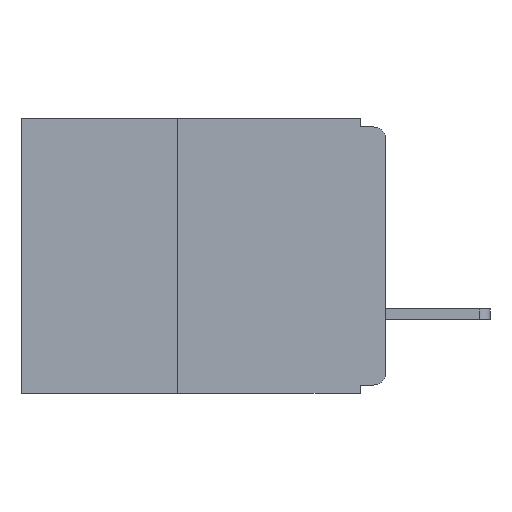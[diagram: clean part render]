
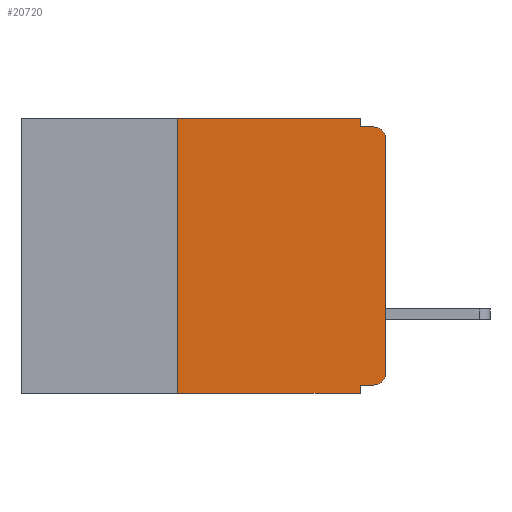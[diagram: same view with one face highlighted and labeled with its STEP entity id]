
A CAD part, left-side view. The second image highlights one B-rep face of the part: STEP entity #20720.
In plain terms, the highlighted planar face has unit normal (-1, 0, 0).
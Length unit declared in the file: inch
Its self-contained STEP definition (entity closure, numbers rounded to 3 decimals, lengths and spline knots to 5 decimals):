
#39 = CARTESIAN_POINT ( 'NONE',  ( 0., 0.031, -0.32 ) ) ;
#455 = ORIENTED_EDGE ( 'NONE', *, *, #13038, .T. ) ;
#470 = CIRCLE ( 'NONE', #14085, 0.015 ) ;
#576 = ORIENTED_EDGE ( 'NONE', *, *, #14436, .F. ) ;
#778 = VERTEX_POINT ( 'NONE', #17617 ) ;
#1560 = DIRECTION ( 'NONE',  ( 1., 0., 0. ) ) ;
#2239 = DIRECTION ( 'NONE',  ( 0., -1., 0. ) ) ;
#2416 = VECTOR ( 'NONE', #14217, 39.37008 ) ;
#2680 = VECTOR ( 'NONE', #23399, 39.37008 ) ;
#3169 = ORIENTED_EDGE ( 'NONE', *, *, #25854, .F. ) ;
#4152 = EDGE_LOOP ( 'NONE', ( #12530, #17470, #6061, #576, #20243, #14952, #4590, #7524, #3169, #455 ) ) ;
#4590 = ORIENTED_EDGE ( 'NONE', *, *, #21514, .T. ) ;
#5326 = CARTESIAN_POINT ( 'NONE',  ( 0., 0.031, -0.01 ) ) ;
#6061 = ORIENTED_EDGE ( 'NONE', *, *, #19302, .F. ) ;
#6496 = EDGE_CURVE ( 'NONE', #16651, #16271, #28083, .T. ) ;
#6736 = EDGE_CURVE ( 'NONE', #778, #7123, #470, .T. ) ;
#7123 = VERTEX_POINT ( 'NONE', #18079 ) ;
#7524 = ORIENTED_EDGE ( 'NONE', *, *, #6496, .F. ) ;
#7761 = VECTOR ( 'NONE', #26527, 39.37008 ) ;
#7963 = DIRECTION ( 'NONE',  ( 0., 0., -1. ) ) ;
#8471 = CARTESIAN_POINT ( 'NONE',  ( 0., 0., -0.01 ) ) ;
#8475 = EDGE_CURVE ( 'NONE', #19391, #31852, #27575, .T. ) ;
#8535 = CARTESIAN_POINT ( 'NONE',  ( 0., 0.015, -0.32 ) ) ;
#8830 = CARTESIAN_POINT ( 'NONE',  ( 0., 0.015, -0.305 ) ) ;
#8921 = CARTESIAN_POINT ( 'NONE',  ( 0., 0.015, -0.025 ) ) ;
#9247 = CARTESIAN_POINT ( 'NONE',  ( 0., 0., 0. ) ) ;
#9705 = CARTESIAN_POINT ( 'NONE',  ( 0., 0.25, 0. ) ) ;
#11346 = DIRECTION ( 'NONE',  ( 0., 0., -1. ) ) ;
#11425 = DIRECTION ( 'NONE',  ( 0., 0., -1. ) ) ;
#12138 = CARTESIAN_POINT ( 'NONE',  ( 0., 0., -0.305 ) ) ;
#12447 = LINE ( 'NONE', #29441, #24897 ) ;
#12530 = ORIENTED_EDGE ( 'NONE', *, *, #26299, .T. ) ;
#13038 = EDGE_CURVE ( 'NONE', #31084, #28289, #14457, .T. ) ;
#14085 = AXIS2_PLACEMENT_3D ( 'NONE', #8921, #26303, #11425 ) ;
#14217 = DIRECTION ( 'NONE',  ( 0., 0., 1. ) ) ;
#14436 = EDGE_CURVE ( 'NONE', #26200, #24440, #17128, .T. ) ;
#14457 = CIRCLE ( 'NONE', #27734, 0.015 ) ;
#14730 = DIRECTION ( 'NONE',  ( 0., -1., 0. ) ) ;
#14875 = LINE ( 'NONE', #29596, #21638 ) ;
#14952 = ORIENTED_EDGE ( 'NONE', *, *, #8475, .F. ) ;
#16020 = CARTESIAN_POINT ( 'NONE',  ( 0., 0.031, 0. ) ) ;
#16253 = AXIS2_PLACEMENT_3D ( 'NONE', #16438, #1560, #19012 ) ;
#16255 = CARTESIAN_POINT ( 'NONE',  ( 0., 0.031, -0.33 ) ) ;
#16271 = VERTEX_POINT ( 'NONE', #16255 ) ;
#16288 = CARTESIAN_POINT ( 'NONE',  ( 0., 0.031, 0. ) ) ;
#16438 = CARTESIAN_POINT ( 'NONE',  ( 0., 0.437, 0. ) ) ;
#16640 = LINE ( 'NONE', #8471, #2680 ) ;
#16651 = VERTEX_POINT ( 'NONE', #39 ) ;
#17128 = LINE ( 'NONE', #16020, #22240 ) ;
#17210 = CARTESIAN_POINT ( 'NONE',  ( 0., 0., -0.32 ) ) ;
#17470 = ORIENTED_EDGE ( 'NONE', *, *, #6736, .T. ) ;
#17617 = CARTESIAN_POINT ( 'NONE',  ( 0., 0., -0.025 ) ) ;
#18079 = CARTESIAN_POINT ( 'NONE',  ( 0., 0.015, -0.01 ) ) ;
#18367 = EDGE_CURVE ( 'NONE', #31852, #26200, #12447, .T. ) ;
#19012 = DIRECTION ( 'NONE',  ( 0., 0., -1. ) ) ;
#19302 = EDGE_CURVE ( 'NONE', #24440, #7123, #16640, .T. ) ;
#19391 = VERTEX_POINT ( 'NONE', #31096 ) ;
#19770 = DIRECTION ( 'NONE',  ( 0., 1., 0. ) ) ;
#20243 = ORIENTED_EDGE ( 'NONE', *, *, #18367, .F. ) ;
#20428 = CARTESIAN_POINT ( 'NONE',  ( 0., 0.031, -0.33 ) ) ;
#20720 = ADVANCED_FACE ( 'NONE', ( #21694 ), #31251, .F. ) ;
#21514 = EDGE_CURVE ( 'NONE', #19391, #16271, #14875, .T. ) ;
#21638 = VECTOR ( 'NONE', #14730, 39.37008 ) ;
#21694 = FACE_OUTER_BOUND ( 'NONE', #4152, .T. ) ;
#22240 = VECTOR ( 'NONE', #25942, 39.37008 ) ;
#23068 = LINE ( 'NONE', #17210, #28806 ) ;
#23399 = DIRECTION ( 'NONE',  ( 0., -1., 0. ) ) ;
#24440 = VERTEX_POINT ( 'NONE', #5326 ) ;
#24897 = VECTOR ( 'NONE', #2239, 39.37008 ) ;
#25854 = EDGE_CURVE ( 'NONE', #31084, #16651, #23068, .T. ) ;
#25942 = DIRECTION ( 'NONE',  ( 0., 0., -1. ) ) ;
#26200 = VERTEX_POINT ( 'NONE', #16288 ) ;
#26213 = DIRECTION ( 'NONE',  ( -1., 0., 0. ) ) ;
#26299 = EDGE_CURVE ( 'NONE', #28289, #778, #28778, .T. ) ;
#26303 = DIRECTION ( 'NONE',  ( -1., 0., 0. ) ) ;
#26527 = DIRECTION ( 'NONE',  ( 0., 0., 1. ) ) ;
#27333 = VECTOR ( 'NONE', #7963, 39.37008 ) ;
#27575 = LINE ( 'NONE', #28868, #7761 ) ;
#27734 = AXIS2_PLACEMENT_3D ( 'NONE', #8830, #26213, #11346 ) ;
#28083 = LINE ( 'NONE', #20428, #27333 ) ;
#28289 = VERTEX_POINT ( 'NONE', #12138 ) ;
#28778 = LINE ( 'NONE', #9247, #2416 ) ;
#28806 = VECTOR ( 'NONE', #19770, 39.37008 ) ;
#28868 = CARTESIAN_POINT ( 'NONE',  ( 0., 0.25, -0.33 ) ) ;
#29441 = CARTESIAN_POINT ( 'NONE',  ( 0., 0.437, 0. ) ) ;
#29596 = CARTESIAN_POINT ( 'NONE',  ( 0., 0.437, -0.33 ) ) ;
#31084 = VERTEX_POINT ( 'NONE', #8535 ) ;
#31096 = CARTESIAN_POINT ( 'NONE',  ( 0., 0.25, -0.33 ) ) ;
#31251 = PLANE ( 'NONE',  #16253 ) ;
#31852 = VERTEX_POINT ( 'NONE', #9705 ) ;
